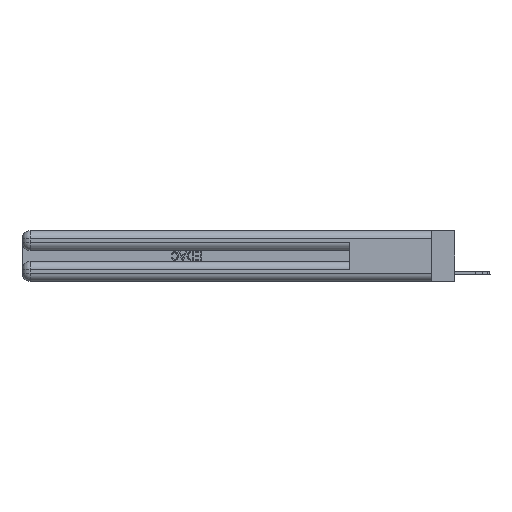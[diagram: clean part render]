
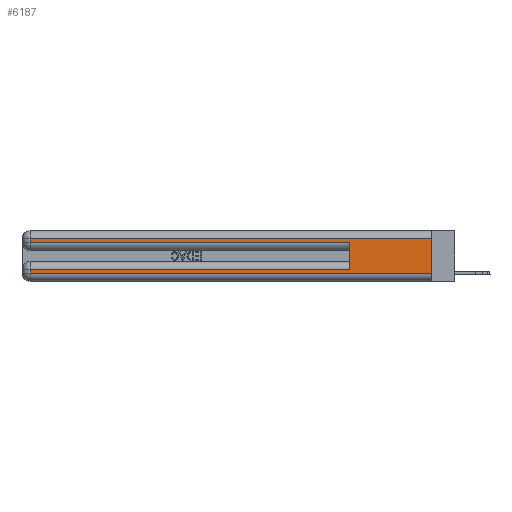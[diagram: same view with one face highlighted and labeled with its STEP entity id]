
A CAD part, left-side view. The second image highlights one B-rep face of the part: STEP entity #6187.
In plain terms, the highlighted planar face has unit normal (-1, 0, 0).
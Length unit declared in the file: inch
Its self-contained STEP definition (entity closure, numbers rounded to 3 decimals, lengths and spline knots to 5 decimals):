
#11 = EDGE_CURVE ( 'NONE', #22372, #4262, #13796, .T. ) ;
#710 = VERTEX_POINT ( 'NONE', #4271 ) ;
#910 = EDGE_LOOP ( 'NONE', ( #3476, #20040, #23773, #25719, #26512, #22612, #6693, #13362 ) ) ;
#1100 = CARTESIAN_POINT ( 'NONE',  ( 0., 2.94, 0.31 ) ) ;
#1178 = AXIS2_PLACEMENT_3D ( 'NONE', #19767, #6142, #6279 ) ;
#2033 = LINE ( 'NONE', #10796, #13446 ) ;
#2289 = DIRECTION ( 'NONE',  ( 0., 1., 0. ) ) ;
#2508 = EDGE_CURVE ( 'NONE', #21850, #710, #2033, .T. ) ;
#3266 = EDGE_CURVE ( 'NONE', #7102, #710, #21237, .T. ) ;
#3476 = ORIENTED_EDGE ( 'NONE', *, *, #2508, .F. ) ;
#3859 = CARTESIAN_POINT ( 'NONE',  ( 0., 0., 0.06 ) ) ;
#4262 = VERTEX_POINT ( 'NONE', #24880 ) ;
#4271 = CARTESIAN_POINT ( 'NONE',  ( 0., 0., 0.06 ) ) ;
#4697 = VERTEX_POINT ( 'NONE', #1100 ) ;
#4753 = LINE ( 'NONE', #24126, #22106 ) ;
#4812 = CARTESIAN_POINT ( 'NONE',  ( 0., 0.6, 0.085 ) ) ;
#5815 = EDGE_CURVE ( 'NONE', #21850, #4697, #21986, .T. ) ;
#5999 = DIRECTION ( 'NONE',  ( 0., -1., 0. ) ) ;
#6142 = DIRECTION ( 'NONE',  ( 1., 0., 0. ) ) ;
#6187 = ADVANCED_FACE ( 'NONE', ( #25676 ), #15174, .F. ) ;
#6279 = DIRECTION ( 'NONE',  ( 0., 0., -1. ) ) ;
#6693 = ORIENTED_EDGE ( 'NONE', *, *, #25039, .T. ) ;
#7102 = VERTEX_POINT ( 'NONE', #23256 ) ;
#7940 = LINE ( 'NONE', #16828, #13312 ) ;
#8460 = VECTOR ( 'NONE', #2289, 39.37008 ) ;
#9454 = VERTEX_POINT ( 'NONE', #4812 ) ;
#9624 = VECTOR ( 'NONE', #20405, 39.37008 ) ;
#9923 = CARTESIAN_POINT ( 'NONE',  ( 0., 2.94, 0.085 ) ) ;
#10796 = CARTESIAN_POINT ( 'NONE',  ( 0., 0., 0.37 ) ) ;
#10820 = VERTEX_POINT ( 'NONE', #9923 ) ;
#11265 = CARTESIAN_POINT ( 'NONE',  ( 0., 2.94, 0.37 ) ) ;
#11367 = CARTESIAN_POINT ( 'NONE',  ( 0., 0., 0.31 ) ) ;
#11654 = CARTESIAN_POINT ( 'NONE',  ( 0., 0., 0.285 ) ) ;
#12590 = EDGE_CURVE ( 'NONE', #4697, #22372, #4753, .T. ) ;
#13208 = EDGE_CURVE ( 'NONE', #9454, #10820, #7940, .T. ) ;
#13312 = VECTOR ( 'NONE', #25206, 39.37008 ) ;
#13362 = ORIENTED_EDGE ( 'NONE', *, *, #3266, .T. ) ;
#13446 = VECTOR ( 'NONE', #20119, 39.37008 ) ;
#13796 = LINE ( 'NONE', #11654, #9624 ) ;
#14031 = CARTESIAN_POINT ( 'NONE',  ( 0., 2.94, 0.285 ) ) ;
#15146 = VECTOR ( 'NONE', #20003, 39.37008 ) ;
#15174 = PLANE ( 'NONE',  #1178 ) ;
#15828 = CARTESIAN_POINT ( 'NONE',  ( 0., 0.6, 0.145 ) ) ;
#16828 = CARTESIAN_POINT ( 'NONE',  ( 0., 0., 0.085 ) ) ;
#17196 = CARTESIAN_POINT ( 'NONE',  ( 0., 0., 0.31 ) ) ;
#18108 = LINE ( 'NONE', #15828, #19257 ) ;
#19257 = VECTOR ( 'NONE', #24481, 39.37008 ) ;
#19767 = CARTESIAN_POINT ( 'NONE',  ( 0., 0., 0.37 ) ) ;
#20003 = DIRECTION ( 'NONE',  ( 0., 0., -1. ) ) ;
#20040 = ORIENTED_EDGE ( 'NONE', *, *, #5815, .T. ) ;
#20119 = DIRECTION ( 'NONE',  ( 0., 0., -1. ) ) ;
#20405 = DIRECTION ( 'NONE',  ( 0., -1., 0. ) ) ;
#21237 = LINE ( 'NONE', #3859, #24963 ) ;
#21850 = VERTEX_POINT ( 'NONE', #11367 ) ;
#21986 = LINE ( 'NONE', #17196, #8460 ) ;
#22106 = VECTOR ( 'NONE', #28255, 39.37008 ) ;
#22188 = LINE ( 'NONE', #11265, #15146 ) ;
#22372 = VERTEX_POINT ( 'NONE', #14031 ) ;
#22612 = ORIENTED_EDGE ( 'NONE', *, *, #13208, .T. ) ;
#23256 = CARTESIAN_POINT ( 'NONE',  ( 0., 2.94, 0.06 ) ) ;
#23773 = ORIENTED_EDGE ( 'NONE', *, *, #12590, .T. ) ;
#24126 = CARTESIAN_POINT ( 'NONE',  ( 0., 2.94, 0.37 ) ) ;
#24481 = DIRECTION ( 'NONE',  ( 0., 0., 1. ) ) ;
#24880 = CARTESIAN_POINT ( 'NONE',  ( 0., 0.6, 0.285 ) ) ;
#24963 = VECTOR ( 'NONE', #5999, 39.37008 ) ;
#24997 = EDGE_CURVE ( 'NONE', #9454, #4262, #18108, .T. ) ;
#25039 = EDGE_CURVE ( 'NONE', #10820, #7102, #22188, .T. ) ;
#25206 = DIRECTION ( 'NONE',  ( 0., 1., 0. ) ) ;
#25676 = FACE_OUTER_BOUND ( 'NONE', #910, .T. ) ;
#25719 = ORIENTED_EDGE ( 'NONE', *, *, #11, .T. ) ;
#26512 = ORIENTED_EDGE ( 'NONE', *, *, #24997, .F. ) ;
#28255 = DIRECTION ( 'NONE',  ( 0., 0., -1. ) ) ;
